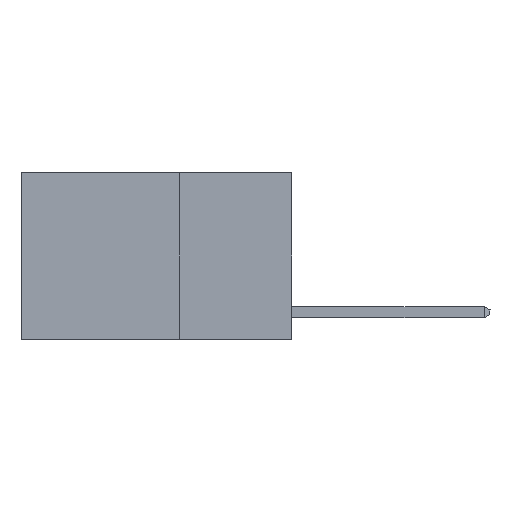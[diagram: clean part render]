
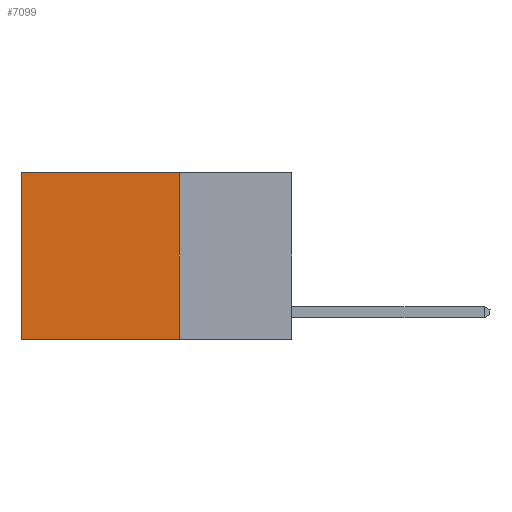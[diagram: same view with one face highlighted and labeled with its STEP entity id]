
A CAD part, left-side view. The second image highlights one B-rep face of the part: STEP entity #7099.
In plain terms, the highlighted planar face has unit normal (-1, 0, 0).
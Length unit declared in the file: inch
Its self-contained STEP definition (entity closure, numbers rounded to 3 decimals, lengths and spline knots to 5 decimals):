
#37 = VECTOR ( 'NONE', #15346, 39.37008 ) ;
#873 = CARTESIAN_POINT ( 'NONE',  ( 0.2625, 0.6, 0. ) ) ;
#1000 = CARTESIAN_POINT ( 'NONE',  ( 0.2625, 0.6, -0.37 ) ) ;
#1225 = PLANE ( 'NONE',  #17719 ) ;
#1798 = VERTEX_POINT ( 'NONE', #1000 ) ;
#3148 = DIRECTION ( 'NONE',  ( 1., 0., 0. ) ) ;
#3734 = ORIENTED_EDGE ( 'NONE', *, *, #18833, .T. ) ;
#3877 = ORIENTED_EDGE ( 'NONE', *, *, #19665, .F. ) ;
#4686 = ORIENTED_EDGE ( 'NONE', *, *, #18517, .F. ) ;
#4808 = VECTOR ( 'NONE', #9178, 39.37008 ) ;
#5143 = LINE ( 'NONE', #13325, #37 ) ;
#6590 = CARTESIAN_POINT ( 'NONE',  ( 0.2625, 0.25, -0.37 ) ) ;
#7011 = VERTEX_POINT ( 'NONE', #6590 ) ;
#7099 = ADVANCED_FACE ( 'NONE', ( #10591 ), #1225, .F. ) ;
#7907 = ORIENTED_EDGE ( 'NONE', *, *, #19447, .T. ) ;
#9111 = EDGE_LOOP ( 'NONE', ( #7907, #4686, #3877, #3734 ) ) ;
#9178 = DIRECTION ( 'NONE',  ( 0., 0., -1. ) ) ;
#9179 = VERTEX_POINT ( 'NONE', #17500 ) ;
#10550 = DIRECTION ( 'NONE',  ( 0., 1., 0. ) ) ;
#10591 = FACE_OUTER_BOUND ( 'NONE', #9111, .T. ) ;
#10612 = DIRECTION ( 'NONE',  ( 0., 0., -1. ) ) ;
#13325 = CARTESIAN_POINT ( 'NONE',  ( 0.2625, 0.25, 0. ) ) ;
#13835 = VECTOR ( 'NONE', #10612, 39.37008 ) ;
#14011 = VERTEX_POINT ( 'NONE', #15373 ) ;
#14473 = CARTESIAN_POINT ( 'NONE',  ( 0.2625, 0.25, -0.37 ) ) ;
#15346 = DIRECTION ( 'NONE',  ( 0., 1., 0. ) ) ;
#15373 = CARTESIAN_POINT ( 'NONE',  ( 0.2625, 0.6, 0. ) ) ;
#17023 = DIRECTION ( 'NONE',  ( 0., 0., -1. ) ) ;
#17500 = CARTESIAN_POINT ( 'NONE',  ( 0.2625, 0.25, 0. ) ) ;
#17719 = AXIS2_PLACEMENT_3D ( 'NONE', #22485, #3148, #17023 ) ;
#18517 = EDGE_CURVE ( 'NONE', #7011, #1798, #21112, .T. ) ;
#18833 = EDGE_CURVE ( 'NONE', #9179, #14011, #5143, .T. ) ;
#19030 = CARTESIAN_POINT ( 'NONE',  ( 0.2625, 0.25, 0. ) ) ;
#19447 = EDGE_CURVE ( 'NONE', #14011, #1798, #24016, .T. ) ;
#19665 = EDGE_CURVE ( 'NONE', #9179, #7011, #20480, .T. ) ;
#20480 = LINE ( 'NONE', #19030, #4808 ) ;
#20522 = VECTOR ( 'NONE', #10550, 39.37008 ) ;
#21112 = LINE ( 'NONE', #14473, #20522 ) ;
#22485 = CARTESIAN_POINT ( 'NONE',  ( 0.2625, 0.25, 0. ) ) ;
#24016 = LINE ( 'NONE', #873, #13835 ) ;
